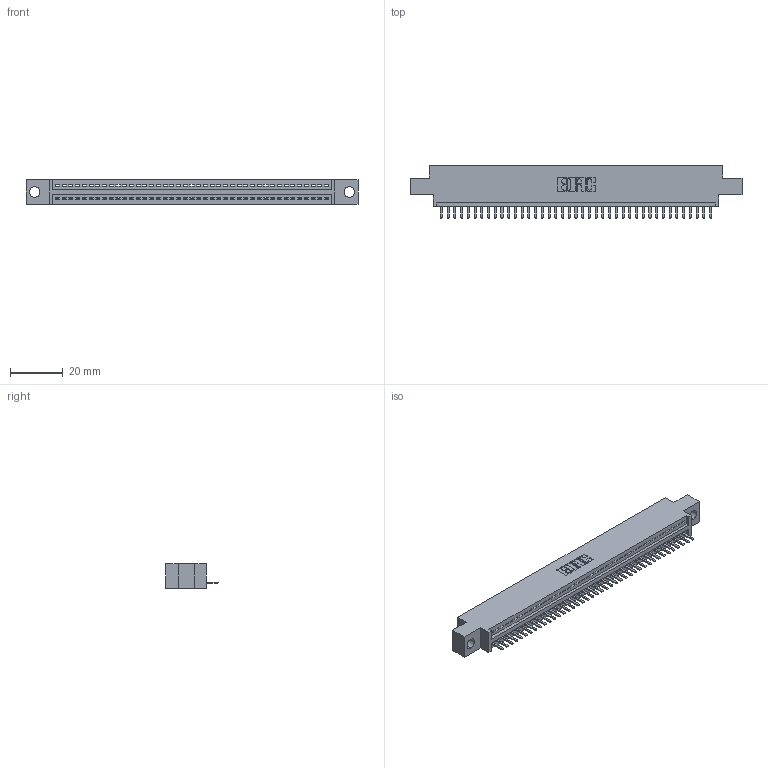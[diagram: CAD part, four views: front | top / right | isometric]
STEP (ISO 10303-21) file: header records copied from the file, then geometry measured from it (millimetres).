
FILE_DESCRIPTION (( 'STEP AP203' ), '1' );
FILE_NAME ('345-041-520-604.STEP', '2021-05-26T14:59:29', ( '' ), ( '' ), 'SwSTEP 2.0', 'SolidWorks 2020', '' );
FILE_SCHEMA (( 'CONFIG_CONTROL_DESIGN' ));
Length unit declared in the file: inch
Products named in the file (3): 345-041-520-604; 345 Part_0.170 Offset - 0.156 Dia-TI; 345-292-001_345-293-120
Assembly tree (42 placements, depth 2):
  345-041-520-604
    345 Part_0.170 Offset - 0.156 Dia-TI
    345-292-001_345-293-120  x41
Bounding box: 125.35 x 19.68 x 9.4 mm (x, y, z)
Volume: 11560.3 mm3; surface area: 14932.2 mm2
Topology: 42 solids, 42 shells, 2686 faces, 7933 edges, 5178 vertices
Faces by surface type: plane 1820, cylinder 866
Entity records: 31657 total; most frequent: CARTESIAN_POINT 5505, ORIENTED_EDGE 5466, DIRECTION 4795, EDGE_CURVE 2733, LINE 2433, VECTOR 2433, VERTEX_POINT 1818, AXIS2_PLACEMENT_3D 1181
